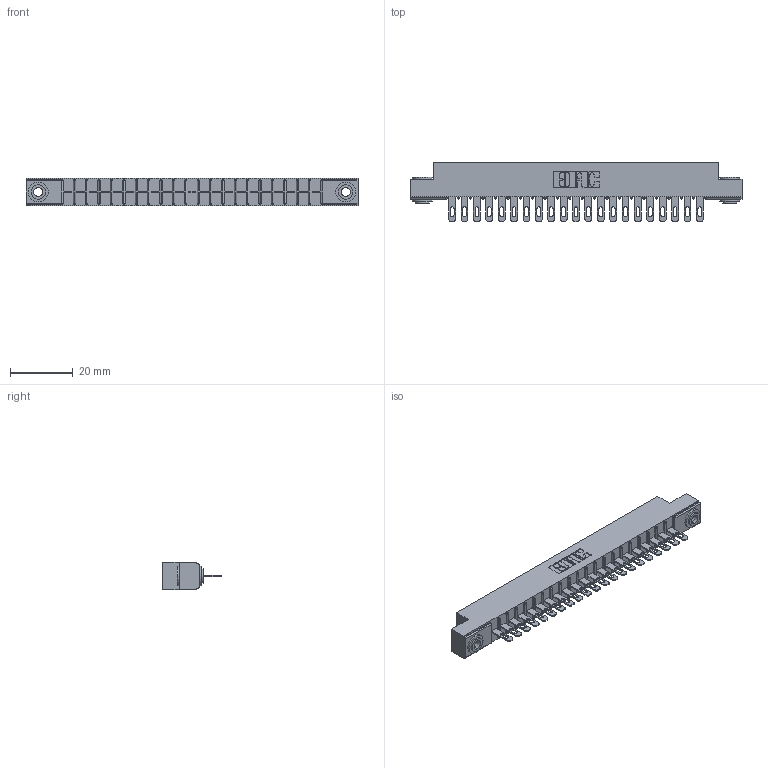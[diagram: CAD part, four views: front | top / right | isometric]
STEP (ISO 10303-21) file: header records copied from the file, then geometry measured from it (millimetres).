
FILE_DESCRIPTION (( 'STEP AP203' ), '1' );
FILE_NAME ('316-021-400-103.STEP', '2020-09-22T19:50:55', ( '' ), ( '' ), 'SwSTEP 2.0', 'SolidWorks 2020', '' );
FILE_SCHEMA (( 'CONFIG_CONTROL_DESIGN' ));
Length unit declared in the file: inch
Products named in the file (4): 345-250-002_345-250-002-102; 306 Part_.156 Dia; 316-021-400-103; 306-290-001_100
Assembly tree (24 placements, depth 2):
  316-021-400-103
    306 Part_.156 Dia
    306-290-001_100  x21
    345-250-002_345-250-002-102  x2
Bounding box: 106.22 x 18.87 x 8.71 mm (x, y, z)
Volume: 7333.2 mm3; surface area: 11388.2 mm2
Topology: 24 solids, 24 shells, 1764 faces, 4943 edges, 3178 vertices
Faces by surface type: plane 1142, cylinder 530, sphere 84, cone 8
Entity records: 23533 total; most frequent: CARTESIAN_POINT 3927, DIRECTION 3889, ORIENTED_EDGE 3882, EDGE_CURVE 1941, LINE 1497, VECTOR 1497, VERTEX_POINT 1234, AXIS2_PLACEMENT_3D 1196
